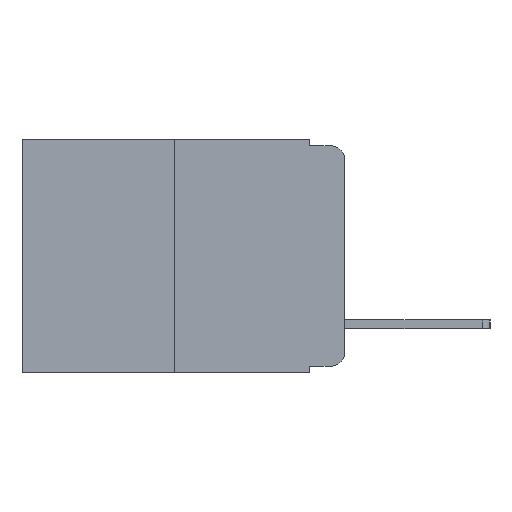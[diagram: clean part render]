
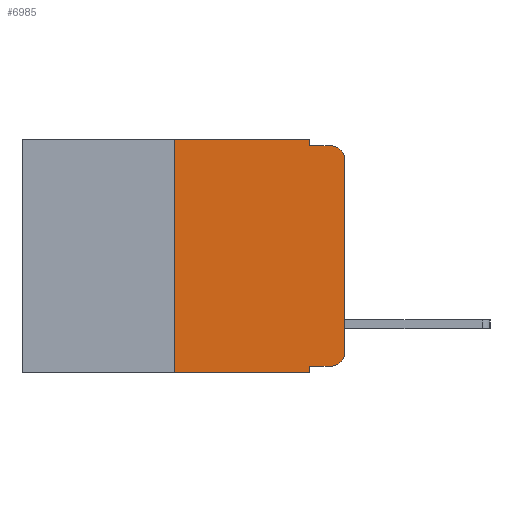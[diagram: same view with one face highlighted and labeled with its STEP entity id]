
A CAD part, left-side view. The second image highlights one B-rep face of the part: STEP entity #6985.
In plain terms, the highlighted planar face has unit normal (-1, 0, 0).
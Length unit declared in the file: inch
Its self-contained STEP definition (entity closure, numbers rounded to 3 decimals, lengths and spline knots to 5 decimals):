
#136 = DIRECTION ( 'NONE',  ( 0., 0., 1. ) ) ;
#227 = CARTESIAN_POINT ( 'NONE',  ( 0., 0.25, 0. ) ) ;
#274 = EDGE_CURVE ( 'NONE', #3873, #9277, #9855, .T. ) ;
#410 = EDGE_CURVE ( 'NONE', #12205, #2598, #7738, .T. ) ;
#438 = VECTOR ( 'NONE', #6681, 39.37008 ) ;
#492 = ORIENTED_EDGE ( 'NONE', *, *, #5708, .F. ) ;
#651 = DIRECTION ( 'NONE',  ( 0., 0., -1. ) ) ;
#716 = LINE ( 'NONE', #8746, #10680 ) ;
#1042 = DIRECTION ( 'NONE',  ( 0., -1., 0. ) ) ;
#1221 = CARTESIAN_POINT ( 'NONE',  ( 0., 0.25, 0. ) ) ;
#1517 = CIRCLE ( 'NONE', #7656, 0.02 ) ;
#1972 = DIRECTION ( 'NONE',  ( 0., -1., 0. ) ) ;
#2017 = CARTESIAN_POINT ( 'NONE',  ( 0., 0.051, -0.333 ) ) ;
#2119 = CARTESIAN_POINT ( 'NONE',  ( 0., 0.051, -0.01 ) ) ;
#2297 = CARTESIAN_POINT ( 'NONE',  ( 0., 0.051, 0. ) ) ;
#2319 = CARTESIAN_POINT ( 'NONE',  ( 0., 0.473, 0. ) ) ;
#2462 = VERTEX_POINT ( 'NONE', #8114 ) ;
#2598 = VERTEX_POINT ( 'NONE', #1221 ) ;
#2748 = DIRECTION ( 'NONE',  ( -1., 0., 0. ) ) ;
#2801 = CARTESIAN_POINT ( 'NONE',  ( 0., 0.02, -0.313 ) ) ;
#2851 = DIRECTION ( 'NONE',  ( 0., 0., -1. ) ) ;
#2876 = VECTOR ( 'NONE', #9761, 39.37008 ) ;
#2906 = EDGE_CURVE ( 'NONE', #10334, #10724, #3025, .T. ) ;
#3025 = LINE ( 'NONE', #2297, #438 ) ;
#3087 = EDGE_CURVE ( 'NONE', #2462, #9780, #1517, .T. ) ;
#3300 = DIRECTION ( 'NONE',  ( 0., -1., 0. ) ) ;
#3604 = LINE ( 'NONE', #9760, #10966 ) ;
#3827 = VERTEX_POINT ( 'NONE', #4022 ) ;
#3873 = VERTEX_POINT ( 'NONE', #10805 ) ;
#3893 = DIRECTION ( 'NONE',  ( 0., 0., -1. ) ) ;
#4022 = CARTESIAN_POINT ( 'NONE',  ( 0., 0.051, 0. ) ) ;
#4097 = VECTOR ( 'NONE', #3300, 39.37008 ) ;
#4406 = EDGE_CURVE ( 'NONE', #11357, #9277, #716, .T. ) ;
#4442 = EDGE_CURVE ( 'NONE', #12205, #10724, #3604, .T. ) ;
#4448 = FACE_OUTER_BOUND ( 'NONE', #11951, .T. ) ;
#4487 = LINE ( 'NONE', #8637, #4785 ) ;
#4785 = VECTOR ( 'NONE', #2851, 39.37008 ) ;
#4874 = ORIENTED_EDGE ( 'NONE', *, *, #3087, .T. ) ;
#4896 = DIRECTION ( 'NONE',  ( 0., 0., 1. ) ) ;
#4960 = CARTESIAN_POINT ( 'NONE',  ( 0., 0.051, -0.343 ) ) ;
#5144 = PLANE ( 'NONE',  #11634 ) ;
#5194 = VECTOR ( 'NONE', #136, 39.37008 ) ;
#5372 = AXIS2_PLACEMENT_3D ( 'NONE', #8729, #8694, #651 ) ;
#5379 = CARTESIAN_POINT ( 'NONE',  ( 0., 0.051, -0.333 ) ) ;
#5448 = EDGE_CURVE ( 'NONE', #9780, #3873, #7082, .T. ) ;
#5685 = ORIENTED_EDGE ( 'NONE', *, *, #5448, .T. ) ;
#5708 = EDGE_CURVE ( 'NONE', #2598, #3827, #9545, .T. ) ;
#6097 = DIRECTION ( 'NONE',  ( 0., 0., -1. ) ) ;
#6317 = ORIENTED_EDGE ( 'NONE', *, *, #4442, .T. ) ;
#6681 = DIRECTION ( 'NONE',  ( 0., 0., -1. ) ) ;
#6747 = CARTESIAN_POINT ( 'NONE',  ( 0., 0., 0. ) ) ;
#6985 = ADVANCED_FACE ( 'NONE', ( #4448 ), #5144, .F. ) ;
#7082 = LINE ( 'NONE', #6747, #11611 ) ;
#7496 = ORIENTED_EDGE ( 'NONE', *, *, #10043, .T. ) ;
#7656 = AXIS2_PLACEMENT_3D ( 'NONE', #2801, #2748, #3893 ) ;
#7738 = LINE ( 'NONE', #227, #5194 ) ;
#8114 = CARTESIAN_POINT ( 'NONE',  ( 0., 0.02, -0.333 ) ) ;
#8637 = CARTESIAN_POINT ( 'NONE',  ( 0., 0.051, 0. ) ) ;
#8694 = DIRECTION ( 'NONE',  ( -1., 0., 0. ) ) ;
#8720 = ORIENTED_EDGE ( 'NONE', *, *, #2906, .F. ) ;
#8729 = CARTESIAN_POINT ( 'NONE',  ( 0., 0.02, -0.03 ) ) ;
#8746 = CARTESIAN_POINT ( 'NONE',  ( 0., 0.051, -0.01 ) ) ;
#8998 = ORIENTED_EDGE ( 'NONE', *, *, #12334, .F. ) ;
#9035 = CARTESIAN_POINT ( 'NONE',  ( 0., 0.473, 0. ) ) ;
#9054 = ORIENTED_EDGE ( 'NONE', *, *, #410, .F. ) ;
#9277 = VERTEX_POINT ( 'NONE', #11487 ) ;
#9545 = LINE ( 'NONE', #2319, #4097 ) ;
#9760 = CARTESIAN_POINT ( 'NONE',  ( 0., 0.473, -0.343 ) ) ;
#9761 = DIRECTION ( 'NONE',  ( 0., -1., 0. ) ) ;
#9780 = VERTEX_POINT ( 'NONE', #10270 ) ;
#9855 = CIRCLE ( 'NONE', #5372, 0.02 ) ;
#10043 = EDGE_CURVE ( 'NONE', #10334, #2462, #10585, .T. ) ;
#10270 = CARTESIAN_POINT ( 'NONE',  ( 0., 0., -0.313 ) ) ;
#10334 = VERTEX_POINT ( 'NONE', #5379 ) ;
#10350 = ORIENTED_EDGE ( 'NONE', *, *, #4406, .F. ) ;
#10585 = LINE ( 'NONE', #2017, #2876 ) ;
#10680 = VECTOR ( 'NONE', #1972, 39.37008 ) ;
#10724 = VERTEX_POINT ( 'NONE', #4960 ) ;
#10805 = CARTESIAN_POINT ( 'NONE',  ( 0., 0., -0.03 ) ) ;
#10966 = VECTOR ( 'NONE', #1042, 39.37008 ) ;
#11099 = CARTESIAN_POINT ( 'NONE',  ( 0., 0.25, -0.343 ) ) ;
#11357 = VERTEX_POINT ( 'NONE', #2119 ) ;
#11487 = CARTESIAN_POINT ( 'NONE',  ( 0., 0.02, -0.01 ) ) ;
#11611 = VECTOR ( 'NONE', #4896, 39.37008 ) ;
#11634 = AXIS2_PLACEMENT_3D ( 'NONE', #9035, #11863, #6097 ) ;
#11810 = ORIENTED_EDGE ( 'NONE', *, *, #274, .T. ) ;
#11863 = DIRECTION ( 'NONE',  ( 1., 0., 0. ) ) ;
#11951 = EDGE_LOOP ( 'NONE', ( #5685, #11810, #10350, #8998, #492, #9054, #6317, #8720, #7496, #4874 ) ) ;
#12205 = VERTEX_POINT ( 'NONE', #11099 ) ;
#12334 = EDGE_CURVE ( 'NONE', #3827, #11357, #4487, .T. ) ;
